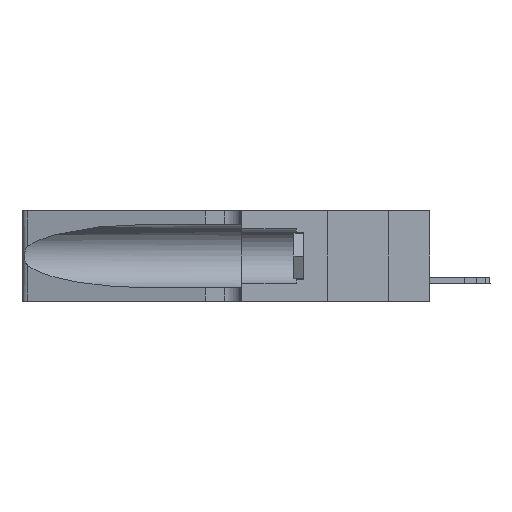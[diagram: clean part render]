
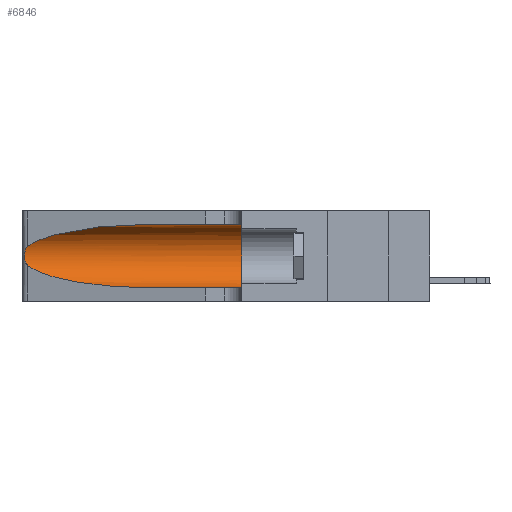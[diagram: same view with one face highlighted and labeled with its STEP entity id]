
A CAD part, left-side view. The second image highlights one B-rep face of the part: STEP entity #6846.
In plain terms, the highlighted cylindrical face has radius 3.308 mm (diameter 6.617 mm), a partial arc.
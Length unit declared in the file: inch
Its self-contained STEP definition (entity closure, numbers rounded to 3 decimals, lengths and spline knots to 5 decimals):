
#870 = CARTESIAN_POINT ( 'NONE',  ( 0.18966, 0.96281, 0.31525 ) ) ;
#1387 = VERTEX_POINT ( 'NONE', #29243 ) ;
#1908 = EDGE_CURVE ( 'NONE', #2691, #15113, #26246, .T. ) ;
#1974 = ORIENTED_EDGE ( 'NONE', *, *, #15339, .F. ) ;
#2250 = ORIENTED_EDGE ( 'NONE', *, *, #16719, .T. ) ;
#2691 = VERTEX_POINT ( 'NONE', #3969 ) ;
#3845 = CARTESIAN_POINT ( 'NONE',  ( 0.26075, 1.23896, 0.19203 ) ) ;
#3969 = CARTESIAN_POINT ( 'NONE',  ( 0.1305, 0.72297, 0.05475 ) ) ;
#4050 = CARTESIAN_POINT ( 'NONE',  ( 0.25639, 1.23184, 0.21858 ) ) ;
#4147 = CARTESIAN_POINT ( 'NONE',  ( 0.26017, 1.23833, 0.17102 ) ) ;
#4268 = AXIS2_PLACEMENT_3D ( 'NONE', #27283, #22649, #8790 ) ;
#4299 = CARTESIAN_POINT ( 'NONE',  ( 0.1305, 0.35, 0.31525 ) ) ;
#5180 = CARTESIAN_POINT ( 'NONE',  ( 0.25487, 1.22718, 0.14631 ) ) ;
#6846 = ADVANCED_FACE ( 'NONE', ( #17447 ), #18532, .F. ) ;
#7649 = CARTESIAN_POINT ( 'NONE',  ( 0.1305, 0.72297, 0.31525 ) ) ;
#7736 = EDGE_CURVE ( 'NONE', #1387, #24861, #19538, .T. ) ;
#7951 = DIRECTION ( 'NONE',  ( 0., -1., 0. ) ) ;
#8232 = CARTESIAN_POINT ( 'NONE',  ( 0.25487, 1.22718, 0.22369 ) ) ;
#8468 = VECTOR ( 'NONE', #7951, 39.37008 ) ;
#8656 = CARTESIAN_POINT ( 'NONE',  ( 0.25856, 1.23593, 0.16098 ) ) ;
#8697 = CARTESIAN_POINT ( 'NONE',  ( 0.1305, 0.72297, 0.05475 ) ) ;
#8757 = CARTESIAN_POINT ( 'NONE',  ( 0.25789, 1.23486, 0.15765 ) ) ;
#8790 = DIRECTION ( 'NONE',  ( 0., 0., -1. ) ) ;
#10307 = CARTESIAN_POINT ( 'NONE',  ( 0.1305, 0.35, 0.05475 ) ) ;
#10590 = VERTEX_POINT ( 'NONE', #7649 ) ;
#10962 = ORIENTED_EDGE ( 'NONE', *, *, #16190, .T. ) ;
#11974 = CARTESIAN_POINT ( 'NONE',  ( 0.1305, 0.72297, 0.31525 ) ) ;
#12818 =( BOUNDED_CURVE ( )  B_SPLINE_CURVE ( 3, ( #29627, #13566, #24900, #8697 ),
 .UNSPECIFIED., .F., .T. ) 
 B_SPLINE_CURVE_WITH_KNOTS ( ( 4, 4 ),
 ( 3.44316, 4.71239 ),
 .UNSPECIFIED. ) 
 CURVE ( )  GEOMETRIC_REPRESENTATION_ITEM ( )  RATIONAL_B_SPLINE_CURVE ( ( 1., 0.87, 0.87, 1. ) ) 
 REPRESENTATION_ITEM ( '' )  );
#12979 = DIRECTION ( 'NONE',  ( 0., -1., 0. ) ) ;
#13316 = CARTESIAN_POINT ( 'NONE',  ( 0.25555, 1.22994, 0.2215 ) ) ;
#13566 = CARTESIAN_POINT ( 'NONE',  ( 0.2373, 1.15595, 0.08982 ) ) ;
#13743 = EDGE_CURVE ( 'NONE', #10590, #16820, #28544, .T. ) ;
#15113 = VERTEX_POINT ( 'NONE', #10307 ) ;
#15339 = EDGE_CURVE ( 'NONE', #16820, #15113, #16796, .T. ) ;
#15548 = CARTESIAN_POINT ( 'NONE',  ( 0.26075, 1.23896, 0.178 ) ) ;
#15759 = CARTESIAN_POINT ( 'NONE',  ( 0.25787, 1.23484, 0.2124 ) ) ;
#16190 = EDGE_CURVE ( 'NONE', #10590, #1387, #23950, .T. ) ;
#16719 = EDGE_CURVE ( 'NONE', #24861, #2691, #12818, .T. ) ;
#16796 = CIRCLE ( 'NONE', #24912, 0.13025 ) ;
#16820 = VERTEX_POINT ( 'NONE', #4299 ) ;
#17447 = FACE_OUTER_BOUND ( 'NONE', #27714, .T. ) ;
#17910 = CARTESIAN_POINT ( 'NONE',  ( 0.26018, 1.23835, 0.19895 ) ) ;
#18532 = CYLINDRICAL_SURFACE ( 'NONE', #4268, 0.13025 ) ;
#19502 = CARTESIAN_POINT ( 'NONE',  ( 0.1305, 1.61858, 0.05475 ) ) ;
#19538 = B_SPLINE_CURVE_WITH_KNOTS ( 'NONE', 3,
 ( #20514, #13316, #4050, #15759, #22829, #17910, #3845, #15548, #4147, #8656, #8757, #25063, #24973, #29481 ),
 .UNSPECIFIED., .F., .F.,
 ( 4, 2, 2, 2, 2, 2, 4 ),
 ( 0., 0.00027, 0.00053, 0.00107, 0.0016, 0.00187, 0.00214 ),
 .UNSPECIFIED. ) ;
#19846 = ORIENTED_EDGE ( 'NONE', *, *, #13743, .F. ) ;
#20514 = CARTESIAN_POINT ( 'NONE',  ( 0.25487, 1.22718, 0.22369 ) ) ;
#21028 = CARTESIAN_POINT ( 'NONE',  ( 0.1305, 0.35, 0.185 ) ) ;
#21586 = VECTOR ( 'NONE', #12979, 39.37008 ) ;
#21982 = CARTESIAN_POINT ( 'NONE',  ( 0.2373, 1.15595, 0.28018 ) ) ;
#21995 = ORIENTED_EDGE ( 'NONE', *, *, #7736, .T. ) ;
#22649 = DIRECTION ( 'NONE',  ( 0., -1., 0. ) ) ;
#22829 = CARTESIAN_POINT ( 'NONE',  ( 0.25854, 1.2359, 0.20912 ) ) ;
#23144 = DIRECTION ( 'NONE',  ( 0., 1., 0. ) ) ;
#23327 = DIRECTION ( 'NONE',  ( 0., 0., 1. ) ) ;
#23950 =( BOUNDED_CURVE ( )  B_SPLINE_CURVE ( 3, ( #11974, #870, #21982, #8232 ),
 .UNSPECIFIED., .F., .F. ) 
 B_SPLINE_CURVE_WITH_KNOTS ( ( 4, 4 ),
 ( 1.5708, 2.84003 ),
 .UNSPECIFIED. ) 
 CURVE ( )  GEOMETRIC_REPRESENTATION_ITEM ( )  RATIONAL_B_SPLINE_CURVE ( ( 1., 0.87, 0.87, 1. ) ) 
 REPRESENTATION_ITEM ( '' )  );
#24861 = VERTEX_POINT ( 'NONE', #5180 ) ;
#24900 = CARTESIAN_POINT ( 'NONE',  ( 0.18966, 0.96281, 0.05475 ) ) ;
#24912 = AXIS2_PLACEMENT_3D ( 'NONE', #21028, #23144, #23327 ) ;
#24973 = CARTESIAN_POINT ( 'NONE',  ( 0.25555, 1.22993, 0.14849 ) ) ;
#25063 = CARTESIAN_POINT ( 'NONE',  ( 0.25639, 1.23186, 0.15144 ) ) ;
#26246 = LINE ( 'NONE', #19502, #8468 ) ;
#27116 = CARTESIAN_POINT ( 'NONE',  ( 0.1305, 1.61858, 0.31525 ) ) ;
#27283 = CARTESIAN_POINT ( 'NONE',  ( 0.1305, 1.61858, 0.185 ) ) ;
#27714 = EDGE_LOOP ( 'NONE', ( #10962, #21995, #2250, #27863, #1974, #19846 ) ) ;
#27863 = ORIENTED_EDGE ( 'NONE', *, *, #1908, .T. ) ;
#28544 = LINE ( 'NONE', #27116, #21586 ) ;
#29243 = CARTESIAN_POINT ( 'NONE',  ( 0.25487, 1.22718, 0.22369 ) ) ;
#29481 = CARTESIAN_POINT ( 'NONE',  ( 0.25487, 1.22718, 0.14631 ) ) ;
#29627 = CARTESIAN_POINT ( 'NONE',  ( 0.25487, 1.22718, 0.14631 ) ) ;
